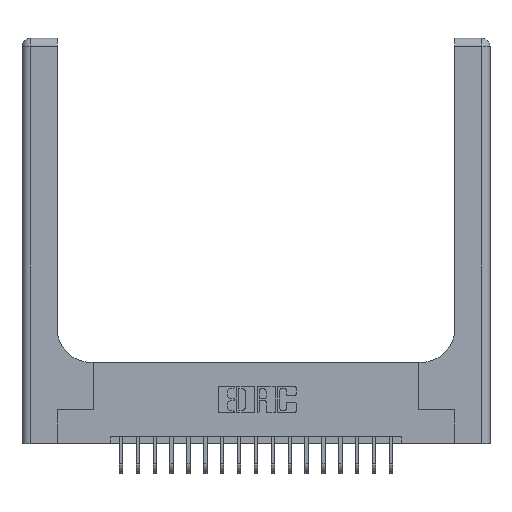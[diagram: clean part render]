
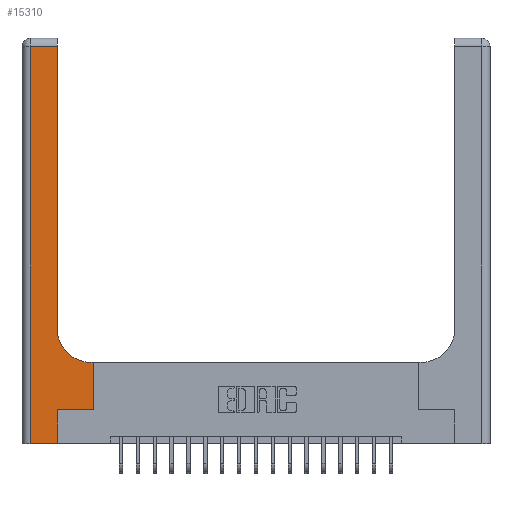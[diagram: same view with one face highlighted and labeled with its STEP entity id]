
A CAD part, top view. The second image highlights one B-rep face of the part: STEP entity #15310.
In plain terms, the highlighted planar face has unit normal (0, 0, 1).
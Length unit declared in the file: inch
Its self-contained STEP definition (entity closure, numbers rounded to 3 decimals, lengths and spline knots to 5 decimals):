
#20 = VERTEX_POINT ( 'NONE', #16168 ) ;
#91 = DIRECTION ( 'NONE',  ( 0., 0., -1. ) ) ;
#493 = VERTEX_POINT ( 'NONE', #14079 ) ;
#1185 = DIRECTION ( 'NONE',  ( 1., 0., 0. ) ) ;
#1690 = DIRECTION ( 'NONE',  ( 0., -1., 0. ) ) ;
#2012 = LINE ( 'NONE', #13429, #21207 ) ;
#2207 = DIRECTION ( 'NONE',  ( -1., 0., 0. ) ) ;
#2235 = ORIENTED_EDGE ( 'NONE', *, *, #12674, .T. ) ;
#2853 = VERTEX_POINT ( 'NONE', #11024 ) ;
#2862 = EDGE_CURVE ( 'NONE', #15799, #4564, #7653, .T. ) ;
#3195 = CARTESIAN_POINT ( 'NONE',  ( 0.26, 2.94, 0.37 ) ) ;
#3205 = VERTEX_POINT ( 'NONE', #20159 ) ;
#3804 = LINE ( 'NONE', #14829, #10820 ) ;
#4095 = CARTESIAN_POINT ( 'NONE',  ( 0., 2.94, 0.37 ) ) ;
#4369 = AXIS2_PLACEMENT_3D ( 'NONE', #10821, #16014, #10964 ) ;
#4564 = VERTEX_POINT ( 'NONE', #7158 ) ;
#4581 = DIRECTION ( 'NONE',  ( 0., 1., 0. ) ) ;
#4671 = CARTESIAN_POINT ( 'NONE',  ( 0.265, 0.25, 0.37 ) ) ;
#5498 = EDGE_CURVE ( 'NONE', #2853, #15513, #19536, .T. ) ;
#6040 = FACE_OUTER_BOUND ( 'NONE', #20876, .T. ) ;
#6129 = EDGE_CURVE ( 'NONE', #11566, #20, #14303, .T. ) ;
#7158 = CARTESIAN_POINT ( 'NONE',  ( 0.265, 0., 0.37 ) ) ;
#7653 = LINE ( 'NONE', #7817, #8689 ) ;
#7725 = LINE ( 'NONE', #12856, #13458 ) ;
#7768 = DIRECTION ( 'NONE',  ( 1., 0., 0. ) ) ;
#7817 = CARTESIAN_POINT ( 'NONE',  ( 0., 0., 0.37 ) ) ;
#8198 = ORIENTED_EDGE ( 'NONE', *, *, #6129, .T. ) ;
#8689 = VECTOR ( 'NONE', #1185, 39.37008 ) ;
#9190 = CARTESIAN_POINT ( 'NONE',  ( 0.06, 0., 0.37 ) ) ;
#9748 = ORIENTED_EDGE ( 'NONE', *, *, #5498, .T. ) ;
#9917 = CIRCLE ( 'NONE', #10744, 0.25 ) ;
#10451 = LINE ( 'NONE', #12129, #21092 ) ;
#10732 = EDGE_CURVE ( 'NONE', #4564, #3205, #7725, .T. ) ;
#10744 = AXIS2_PLACEMENT_3D ( 'NONE', #18304, #91, #11666 ) ;
#10820 = VECTOR ( 'NONE', #1690, 39.37008 ) ;
#10821 = CARTESIAN_POINT ( 'NONE',  ( 0., 3., 0.37 ) ) ;
#10890 = ORIENTED_EDGE ( 'NONE', *, *, #16207, .T. ) ;
#10964 = DIRECTION ( 'NONE',  ( -1., 0., 0. ) ) ;
#11024 = CARTESIAN_POINT ( 'NONE',  ( 0.528, 0.25, 0.37 ) ) ;
#11060 = ORIENTED_EDGE ( 'NONE', *, *, #2862, .T. ) ;
#11176 = ORIENTED_EDGE ( 'NONE', *, *, #11559, .T. ) ;
#11210 = VECTOR ( 'NONE', #11582, 39.37008 ) ;
#11559 = EDGE_CURVE ( 'NONE', #20, #15799, #3804, .T. ) ;
#11566 = VERTEX_POINT ( 'NONE', #3195 ) ;
#11582 = DIRECTION ( 'NONE',  ( 0., 1., 0. ) ) ;
#11584 = EDGE_CURVE ( 'NONE', #15513, #13054, #2012, .T. ) ;
#11666 = DIRECTION ( 'NONE',  ( 1., 0., 0. ) ) ;
#12129 = CARTESIAN_POINT ( 'NONE',  ( 0.26, 3., 0.37 ) ) ;
#12220 = VECTOR ( 'NONE', #2207, 39.37008 ) ;
#12674 = EDGE_CURVE ( 'NONE', #3205, #2853, #19131, .T. ) ;
#12856 = CARTESIAN_POINT ( 'NONE',  ( 0.265, 0., 0.37 ) ) ;
#12994 = ORIENTED_EDGE ( 'NONE', *, *, #11584, .T. ) ;
#13054 = VERTEX_POINT ( 'NONE', #20747 ) ;
#13204 = DIRECTION ( 'NONE',  ( -1., 0., 0. ) ) ;
#13429 = CARTESIAN_POINT ( 'NONE',  ( 0.26, 0.6, 0.37 ) ) ;
#13458 = VECTOR ( 'NONE', #4581, 39.37008 ) ;
#14079 = CARTESIAN_POINT ( 'NONE',  ( 0.26, 0.85, 0.37 ) ) ;
#14291 = ORIENTED_EDGE ( 'NONE', *, *, #10732, .T. ) ;
#14303 = LINE ( 'NONE', #4095, #12220 ) ;
#14735 = ORIENTED_EDGE ( 'NONE', *, *, #15230, .T. ) ;
#14829 = CARTESIAN_POINT ( 'NONE',  ( 0.06, 3., 0.37 ) ) ;
#15230 = EDGE_CURVE ( 'NONE', #493, #11566, #10451, .T. ) ;
#15310 = ADVANCED_FACE ( 'NONE', ( #6040 ), #17655, .F. ) ;
#15372 = DIRECTION ( 'NONE',  ( 0., 1., 0. ) ) ;
#15513 = VERTEX_POINT ( 'NONE', #16085 ) ;
#15799 = VERTEX_POINT ( 'NONE', #9190 ) ;
#16014 = DIRECTION ( 'NONE',  ( 0., 0., -1. ) ) ;
#16085 = CARTESIAN_POINT ( 'NONE',  ( 0.528, 0.6, 0.37 ) ) ;
#16168 = CARTESIAN_POINT ( 'NONE',  ( 0.06, 2.94, 0.37 ) ) ;
#16207 = EDGE_CURVE ( 'NONE', #13054, #493, #9917, .T. ) ;
#16544 = CARTESIAN_POINT ( 'NONE',  ( 0.528, 0.25, 0.37 ) ) ;
#17655 = PLANE ( 'NONE',  #4369 ) ;
#17849 = VECTOR ( 'NONE', #7768, 39.37008 ) ;
#18304 = CARTESIAN_POINT ( 'NONE',  ( 0.51, 0.85, 0.37 ) ) ;
#19131 = LINE ( 'NONE', #4671, #17849 ) ;
#19536 = LINE ( 'NONE', #16544, #11210 ) ;
#20159 = CARTESIAN_POINT ( 'NONE',  ( 0.265, 0.25, 0.37 ) ) ;
#20747 = CARTESIAN_POINT ( 'NONE',  ( 0.51, 0.6, 0.37 ) ) ;
#20876 = EDGE_LOOP ( 'NONE', ( #14735, #8198, #11176, #11060, #14291, #2235, #9748, #12994, #10890 ) ) ;
#21092 = VECTOR ( 'NONE', #15372, 39.37008 ) ;
#21207 = VECTOR ( 'NONE', #13204, 39.37008 ) ;
